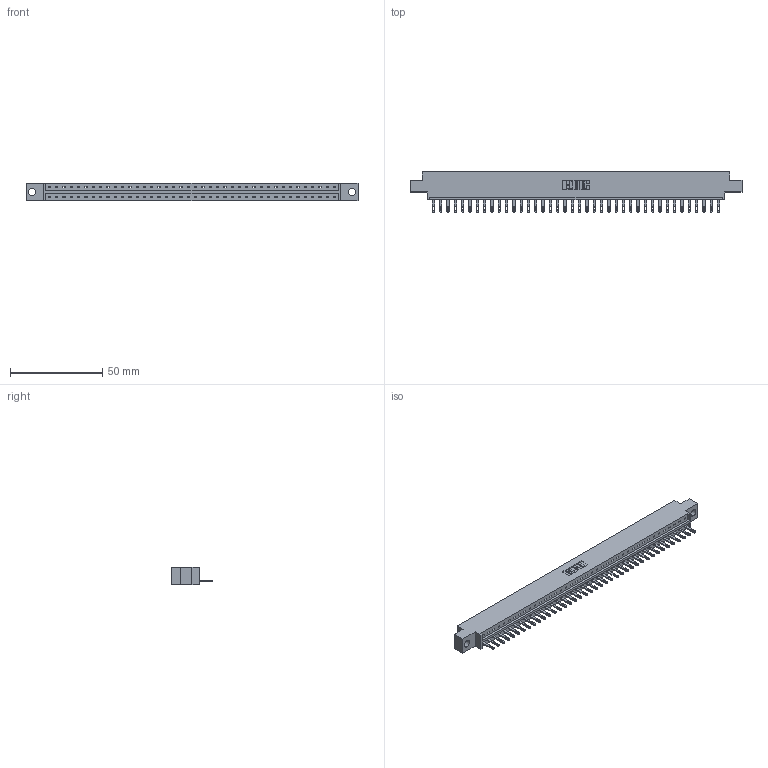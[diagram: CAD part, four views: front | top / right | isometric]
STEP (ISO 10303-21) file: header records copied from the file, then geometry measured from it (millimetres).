
FILE_DESCRIPTION (( 'STEP AP203' ), '1' );
FILE_NAME ('333-040-500-604.STEP', '2018-08-03T13:24:52', ( '' ), ( '' ), 'SwSTEP 2.0', 'SolidWorks 2016', '' );
FILE_SCHEMA (( 'CONFIG_CONTROL_DESIGN' ));
Length unit declared in the file: inch
Products named in the file (3): 333 Part_Offset - .156 Dia - TH; 345-292-001_345-293-100; 333-040-500-604
Assembly tree (41 placements, depth 2):
  333-040-500-604
    333 Part_Offset - .156 Dia - TH
    345-292-001_345-293-100  x40
Bounding box: 180.04 x 21.85 x 9.4 mm (x, y, z)
Volume: 17808.5 mm3; surface area: 19346 mm2
Topology: 41 solids, 41 shells, 2278 faces, 7043 edges, 4694 vertices
Faces by surface type: plane 1514, cylinder 764
Entity records: 24777 total; most frequent: CARTESIAN_POINT 4282, ORIENTED_EDGE 4258, DIRECTION 3617, EDGE_CURVE 2129, LINE 1997, VECTOR 1997, VERTEX_POINT 1418, AXIS2_PLACEMENT_3D 810
